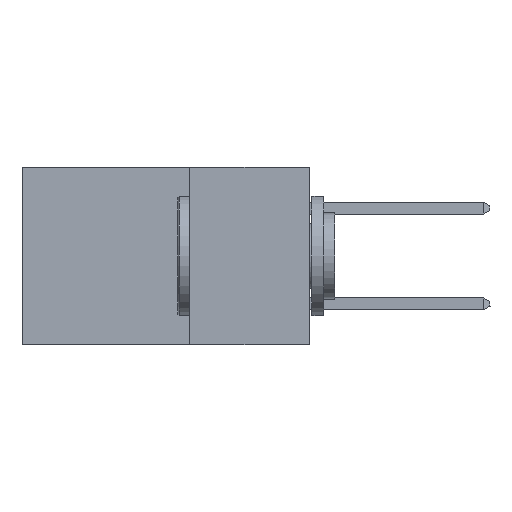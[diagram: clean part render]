
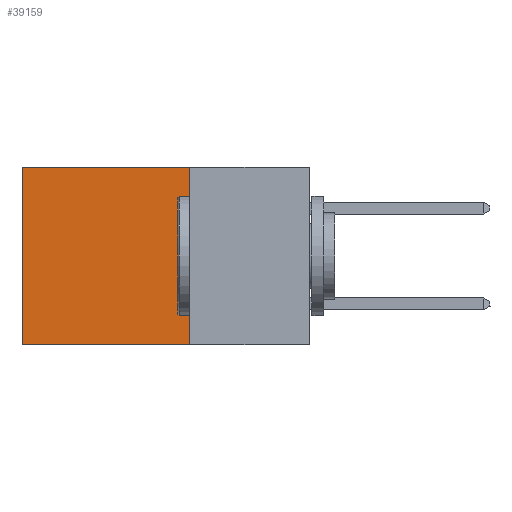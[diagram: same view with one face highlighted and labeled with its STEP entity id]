
A CAD part, left-side view. The second image highlights one B-rep face of the part: STEP entity #39159.
In plain terms, the highlighted planar face has unit normal (-1, 0, 0).
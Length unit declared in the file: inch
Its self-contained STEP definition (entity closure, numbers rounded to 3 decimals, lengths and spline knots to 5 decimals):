
#554 = CARTESIAN_POINT ( 'NONE',  ( 0.2875, 0.25, 0. ) ) ;
#1111 = CARTESIAN_POINT ( 'NONE',  ( 0.2875, 0.25, 0. ) ) ;
#4243 = FACE_OUTER_BOUND ( 'NONE', #13068, .T. ) ;
#4707 = EDGE_CURVE ( 'NONE', #5993, #10416, #41782, .T. ) ;
#5305 = VERTEX_POINT ( 'NONE', #29809 ) ;
#5993 = VERTEX_POINT ( 'NONE', #1111 ) ;
#6929 = DIRECTION ( 'NONE',  ( 0., 0., -1. ) ) ;
#9193 = DIRECTION ( 'NONE',  ( 0., 0., -1. ) ) ;
#9619 = LINE ( 'NONE', #16209, #41951 ) ;
#10416 = VERTEX_POINT ( 'NONE', #31897 ) ;
#11616 = VECTOR ( 'NONE', #36337, 39.37008 ) ;
#11751 = VERTEX_POINT ( 'NONE', #27915 ) ;
#12573 = ORIENTED_EDGE ( 'NONE', *, *, #39647, .T. ) ;
#13068 = EDGE_LOOP ( 'NONE', ( #12573, #40209, #16041, #38208 ) ) ;
#16041 = ORIENTED_EDGE ( 'NONE', *, *, #16266, .F. ) ;
#16209 = CARTESIAN_POINT ( 'NONE',  ( 0.2875, 0.25, -0.37 ) ) ;
#16266 = EDGE_CURVE ( 'NONE', #5993, #5305, #28951, .T. ) ;
#17174 = VECTOR ( 'NONE', #18510, 39.37008 ) ;
#18510 = DIRECTION ( 'NONE',  ( 0., 1., 0. ) ) ;
#22280 = CARTESIAN_POINT ( 'NONE',  ( 0.2875, 0.6, 0. ) ) ;
#22594 = CARTESIAN_POINT ( 'NONE',  ( 0.2875, 0.25, 0. ) ) ;
#22666 = DIRECTION ( 'NONE',  ( 0., 1., 0. ) ) ;
#25194 = CARTESIAN_POINT ( 'NONE',  ( 0.2875, 0.25, 0. ) ) ;
#25966 = DIRECTION ( 'NONE',  ( 1., 0., 0. ) ) ;
#26599 = LINE ( 'NONE', #22280, #34076 ) ;
#27915 = CARTESIAN_POINT ( 'NONE',  ( 0.2875, 0.6, -0.37 ) ) ;
#28951 = LINE ( 'NONE', #554, #11616 ) ;
#29809 = CARTESIAN_POINT ( 'NONE',  ( 0.2875, 0.25, -0.37 ) ) ;
#31897 = CARTESIAN_POINT ( 'NONE',  ( 0.2875, 0.6, 0. ) ) ;
#33027 = AXIS2_PLACEMENT_3D ( 'NONE', #22594, #25966, #6929 ) ;
#34076 = VECTOR ( 'NONE', #9193, 39.37008 ) ;
#36337 = DIRECTION ( 'NONE',  ( 0., 0., -1. ) ) ;
#36815 = EDGE_CURVE ( 'NONE', #5305, #11751, #9619, .T. ) ;
#38208 = ORIENTED_EDGE ( 'NONE', *, *, #4707, .T. ) ;
#38660 = PLANE ( 'NONE',  #33027 ) ;
#39159 = ADVANCED_FACE ( 'NONE', ( #4243 ), #38660, .F. ) ;
#39647 = EDGE_CURVE ( 'NONE', #10416, #11751, #26599, .T. ) ;
#40209 = ORIENTED_EDGE ( 'NONE', *, *, #36815, .F. ) ;
#41782 = LINE ( 'NONE', #25194, #17174 ) ;
#41951 = VECTOR ( 'NONE', #22666, 39.37008 ) ;
